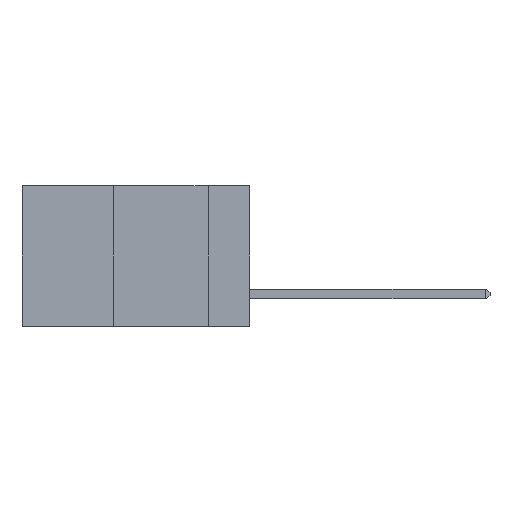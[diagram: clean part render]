
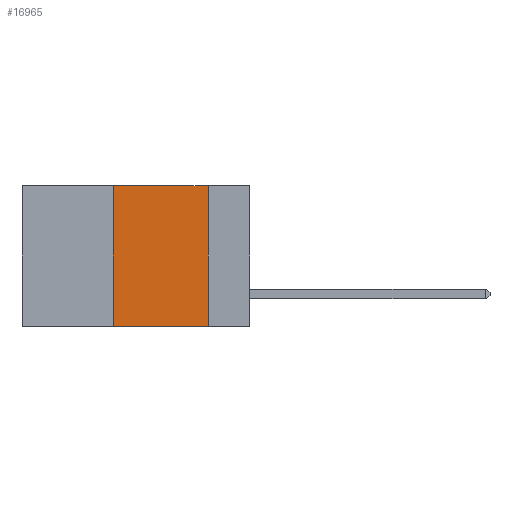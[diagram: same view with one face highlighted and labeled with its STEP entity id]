
A CAD part, left-side view. The second image highlights one B-rep face of the part: STEP entity #16965.
In plain terms, the highlighted planar face has unit normal (-1, 0, 0).
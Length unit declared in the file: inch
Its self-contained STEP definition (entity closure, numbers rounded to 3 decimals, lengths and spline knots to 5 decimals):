
#642 = LINE ( 'NONE', #17623, #34772 ) ;
#2743 = CARTESIAN_POINT ( 'NONE',  ( 0., 0.6, 0. ) ) ;
#4704 = DIRECTION ( 'NONE',  ( 0., 0., -1. ) ) ;
#5490 = LINE ( 'NONE', #37250, #28643 ) ;
#5560 = ORIENTED_EDGE ( 'NONE', *, *, #15249, .T. ) ;
#8439 = DIRECTION ( 'NONE',  ( 0., -1., 0. ) ) ;
#8803 = EDGE_CURVE ( 'NONE', #39614, #26398, #30955, .T. ) ;
#12431 = EDGE_LOOP ( 'NONE', ( #34947, #27276, #13163, #5560 ) ) ;
#12478 = DIRECTION ( 'NONE',  ( 0., -1., 0. ) ) ;
#13060 = CARTESIAN_POINT ( 'NONE',  ( 0., 0.6, 0. ) ) ;
#13163 = ORIENTED_EDGE ( 'NONE', *, *, #30293, .F. ) ;
#13259 = CARTESIAN_POINT ( 'NONE',  ( 0., 0.36, 0. ) ) ;
#15249 = EDGE_CURVE ( 'NONE', #16478, #38520, #5490, .T. ) ;
#16478 = VERTEX_POINT ( 'NONE', #29314 ) ;
#16888 = AXIS2_PLACEMENT_3D ( 'NONE', #2743, #25183, #19018 ) ;
#16965 = ADVANCED_FACE ( 'NONE', ( #28441 ), #28309, .F. ) ;
#17623 = CARTESIAN_POINT ( 'NONE',  ( 0., 0.11, 0. ) ) ;
#19018 = DIRECTION ( 'NONE',  ( 0., 0., -1. ) ) ;
#22366 = VECTOR ( 'NONE', #12478, 39.37008 ) ;
#25183 = DIRECTION ( 'NONE',  ( 1., 0., 0. ) ) ;
#26398 = VERTEX_POINT ( 'NONE', #38139 ) ;
#27276 = ORIENTED_EDGE ( 'NONE', *, *, #8803, .F. ) ;
#28309 = PLANE ( 'NONE',  #16888 ) ;
#28441 = FACE_OUTER_BOUND ( 'NONE', #12431, .T. ) ;
#28643 = VECTOR ( 'NONE', #8439, 39.37008 ) ;
#29314 = CARTESIAN_POINT ( 'NONE',  ( 0., 0.36, -0.37 ) ) ;
#29574 = CARTESIAN_POINT ( 'NONE',  ( 0., 0.36, 0. ) ) ;
#30293 = EDGE_CURVE ( 'NONE', #16478, #39614, #36615, .T. ) ;
#30955 = LINE ( 'NONE', #13060, #22366 ) ;
#32638 = DIRECTION ( 'NONE',  ( 0., 0., 1. ) ) ;
#34772 = VECTOR ( 'NONE', #4704, 39.37008 ) ;
#34947 = ORIENTED_EDGE ( 'NONE', *, *, #39786, .F. ) ;
#36615 = LINE ( 'NONE', #13259, #39635 ) ;
#37250 = CARTESIAN_POINT ( 'NONE',  ( 0., 0.6, -0.37 ) ) ;
#38139 = CARTESIAN_POINT ( 'NONE',  ( 0., 0.11, 0. ) ) ;
#38520 = VERTEX_POINT ( 'NONE', #38820 ) ;
#38820 = CARTESIAN_POINT ( 'NONE',  ( 0., 0.11, -0.37 ) ) ;
#39614 = VERTEX_POINT ( 'NONE', #29574 ) ;
#39635 = VECTOR ( 'NONE', #32638, 39.37008 ) ;
#39786 = EDGE_CURVE ( 'NONE', #26398, #38520, #642, .T. ) ;
